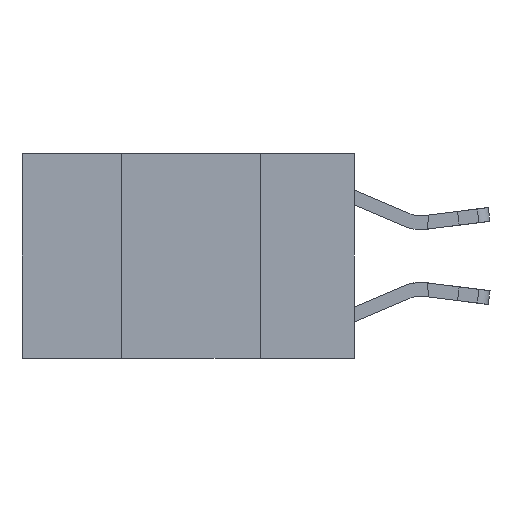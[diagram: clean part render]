
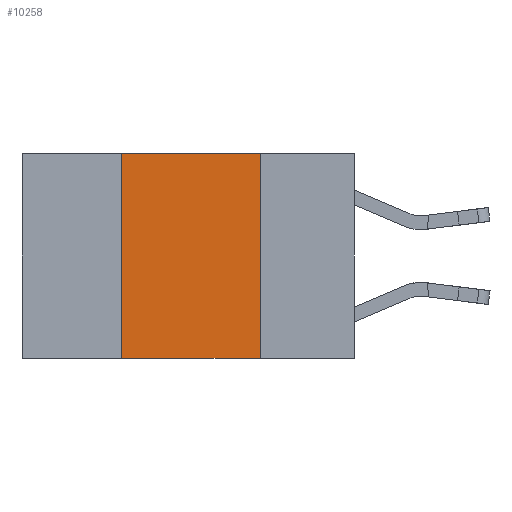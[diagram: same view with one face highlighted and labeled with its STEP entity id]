
A CAD part, left-side view. The second image highlights one B-rep face of the part: STEP entity #10258.
In plain terms, the highlighted planar face has unit normal (-1, 0, 0).
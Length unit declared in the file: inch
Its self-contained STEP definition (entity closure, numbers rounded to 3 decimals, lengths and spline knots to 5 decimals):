
#331 = EDGE_CURVE ( 'NONE', #2332, #21090, #21228, .T. ) ;
#1059 = ORIENTED_EDGE ( 'NONE', *, *, #17936, .F. ) ;
#1497 = ORIENTED_EDGE ( 'NONE', *, *, #6197, .T. ) ;
#2332 = VERTEX_POINT ( 'NONE', #16499 ) ;
#3421 = EDGE_CURVE ( 'NONE', #18247, #2332, #3860, .T. ) ;
#3860 = LINE ( 'NONE', #10453, #5075 ) ;
#4196 = CARTESIAN_POINT ( 'NONE',  ( 0., 0.17, 0. ) ) ;
#4212 = LINE ( 'NONE', #9210, #18298 ) ;
#4415 = CARTESIAN_POINT ( 'NONE',  ( 0., 0.17, -0.37 ) ) ;
#5075 = VECTOR ( 'NONE', #15136, 39.37008 ) ;
#5701 = ORIENTED_EDGE ( 'NONE', *, *, #331, .F. ) ;
#6197 = EDGE_CURVE ( 'NONE', #18247, #9104, #4212, .T. ) ;
#6505 = CARTESIAN_POINT ( 'NONE',  ( 0., 0.17, 0. ) ) ;
#8460 = PLANE ( 'NONE',  #13636 ) ;
#8524 = ORIENTED_EDGE ( 'NONE', *, *, #3421, .F. ) ;
#9104 = VERTEX_POINT ( 'NONE', #4415 ) ;
#9210 = CARTESIAN_POINT ( 'NONE',  ( 0., 0.6, -0.37 ) ) ;
#9790 = VECTOR ( 'NONE', #15571, 39.37008 ) ;
#9864 = CARTESIAN_POINT ( 'NONE',  ( 0., 0.6, 0. ) ) ;
#10072 = CARTESIAN_POINT ( 'NONE',  ( 0., 0.6, 0. ) ) ;
#10258 = ADVANCED_FACE ( 'NONE', ( #13656 ), #8460, .F. ) ;
#10453 = CARTESIAN_POINT ( 'NONE',  ( 0., 0.42, 0. ) ) ;
#13345 = DIRECTION ( 'NONE',  ( 0., -1., 0. ) ) ;
#13553 = DIRECTION ( 'NONE',  ( 0., 0., -1. ) ) ;
#13636 = AXIS2_PLACEMENT_3D ( 'NONE', #10072, #16662, #13553 ) ;
#13656 = FACE_OUTER_BOUND ( 'NONE', #20482, .T. ) ;
#13756 = DIRECTION ( 'NONE',  ( 0., -1., 0. ) ) ;
#15136 = DIRECTION ( 'NONE',  ( 0., 0., 1. ) ) ;
#15571 = DIRECTION ( 'NONE',  ( 0., 0., -1. ) ) ;
#15670 = LINE ( 'NONE', #4196, #9790 ) ;
#16499 = CARTESIAN_POINT ( 'NONE',  ( 0., 0.42, 0. ) ) ;
#16662 = DIRECTION ( 'NONE',  ( 1., 0., 0. ) ) ;
#17936 = EDGE_CURVE ( 'NONE', #21090, #9104, #15670, .T. ) ;
#18247 = VERTEX_POINT ( 'NONE', #18665 ) ;
#18298 = VECTOR ( 'NONE', #13756, 39.37008 ) ;
#18665 = CARTESIAN_POINT ( 'NONE',  ( 0., 0.42, -0.37 ) ) ;
#19758 = VECTOR ( 'NONE', #13345, 39.37008 ) ;
#20482 = EDGE_LOOP ( 'NONE', ( #1059, #5701, #8524, #1497 ) ) ;
#21090 = VERTEX_POINT ( 'NONE', #6505 ) ;
#21228 = LINE ( 'NONE', #9864, #19758 ) ;
